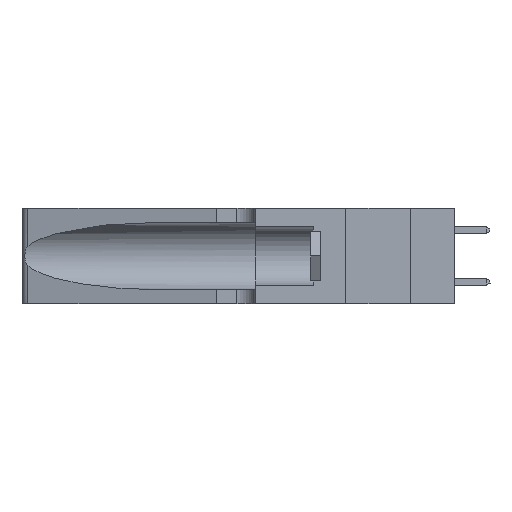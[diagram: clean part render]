
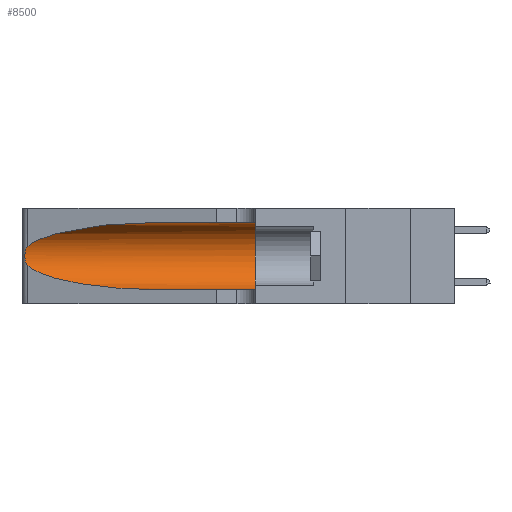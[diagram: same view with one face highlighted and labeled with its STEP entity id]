
A CAD part, left-side view. The second image highlights one B-rep face of the part: STEP entity #8500.
In plain terms, the highlighted cylindrical face has radius 3.308 mm (diameter 6.617 mm), a partial arc.
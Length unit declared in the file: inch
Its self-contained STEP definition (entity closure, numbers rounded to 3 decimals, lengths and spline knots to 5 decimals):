
#525 = CARTESIAN_POINT ( 'NONE',  ( 0.2373, 1.15595, 0.08982 ) ) ;
#903 = EDGE_CURVE ( 'NONE', #39769, #9896, #15293, .T. ) ;
#2294 = EDGE_CURVE ( 'NONE', #9896, #13112, #42863, .T. ) ;
#2593 = CARTESIAN_POINT ( 'NONE',  ( 0.1305, 0.35, 0.31525 ) ) ;
#2891 = EDGE_LOOP ( 'NONE', ( #29773, #40669, #41727, #10534, #13680, #7924 ) ) ;
#3011 = CARTESIAN_POINT ( 'NONE',  ( 0.25856, 1.23593, 0.16098 ) ) ;
#3863 = CARTESIAN_POINT ( 'NONE',  ( 0.1305, 0.72297, 0.05475 ) ) ;
#4471 = VECTOR ( 'NONE', #37388, 39.37008 ) ;
#4519 = AXIS2_PLACEMENT_3D ( 'NONE', #41123, #21231, #24622 ) ;
#4777 = FACE_OUTER_BOUND ( 'NONE', #2891, .T. ) ;
#4916 = CARTESIAN_POINT ( 'NONE',  ( 0.1305, 0.72297, 0.05475 ) ) ;
#6243 = CARTESIAN_POINT ( 'NONE',  ( 0.25487, 1.22718, 0.22369 ) ) ;
#6380 = CARTESIAN_POINT ( 'NONE',  ( 0.25639, 1.23186, 0.15144 ) ) ;
#7137 = DIRECTION ( 'NONE',  ( 0., -1., 0. ) ) ;
#7431 = CARTESIAN_POINT ( 'NONE',  ( 0.1305, 1.61858, 0.31525 ) ) ;
#7924 = ORIENTED_EDGE ( 'NONE', *, *, #27173, .F. ) ;
#8186 = EDGE_CURVE ( 'NONE', #14373, #39769, #42957, .T. ) ;
#8500 = ADVANCED_FACE ( 'NONE', ( #4777 ), #12662, .F. ) ;
#9625 = CARTESIAN_POINT ( 'NONE',  ( 0.25555, 1.22994, 0.2215 ) ) ;
#9757 = CARTESIAN_POINT ( 'NONE',  ( 0.25487, 1.22718, 0.14631 ) ) ;
#9896 = VERTEX_POINT ( 'NONE', #4916 ) ;
#10534 = ORIENTED_EDGE ( 'NONE', *, *, #2294, .T. ) ;
#12099 =( BOUNDED_CURVE ( )  B_SPLINE_CURVE ( 3, ( #35164, #38493, #18640, #41851 ),
 .UNSPECIFIED., .F., .F. ) 
 B_SPLINE_CURVE_WITH_KNOTS ( ( 4, 4 ),
 ( 1.5708, 2.84003 ),
 .UNSPECIFIED. ) 
 CURVE ( )  GEOMETRIC_REPRESENTATION_ITEM ( )  RATIONAL_B_SPLINE_CURVE ( ( 1., 0.87, 0.87, 1. ) ) 
 REPRESENTATION_ITEM ( '' )  );
#12662 = CYLINDRICAL_SURFACE ( 'NONE', #4519, 0.13025 ) ;
#12986 = CARTESIAN_POINT ( 'NONE',  ( 0.25639, 1.23184, 0.21858 ) ) ;
#13112 = VERTEX_POINT ( 'NONE', #34174 ) ;
#13680 = ORIENTED_EDGE ( 'NONE', *, *, #14604, .F. ) ;
#13877 = CARTESIAN_POINT ( 'NONE',  ( 0.1305, 1.61858, 0.05475 ) ) ;
#14373 = VERTEX_POINT ( 'NONE', #19945 ) ;
#14604 = EDGE_CURVE ( 'NONE', #42783, #13112, #31047, .T. ) ;
#15293 =( BOUNDED_CURVE ( )  B_SPLINE_CURVE ( 3, ( #40389, #525, #20532, #3863 ),
 .UNSPECIFIED., .F., .T. ) 
 B_SPLINE_CURVE_WITH_KNOTS ( ( 4, 4 ),
 ( 3.44316, 4.71239 ),
 .UNSPECIFIED. ) 
 CURVE ( )  GEOMETRIC_REPRESENTATION_ITEM ( )  RATIONAL_B_SPLINE_CURVE ( ( 1., 0.87, 0.87, 1. ) ) 
 REPRESENTATION_ITEM ( '' )  );
#16332 = CARTESIAN_POINT ( 'NONE',  ( 0.25854, 1.2359, 0.20912 ) ) ;
#17746 = CARTESIAN_POINT ( 'NONE',  ( 0.1305, 0.35, 0.185 ) ) ;
#18640 = CARTESIAN_POINT ( 'NONE',  ( 0.2373, 1.15595, 0.28018 ) ) ;
#19666 = CARTESIAN_POINT ( 'NONE',  ( 0.26075, 1.23896, 0.19203 ) ) ;
#19945 = CARTESIAN_POINT ( 'NONE',  ( 0.25487, 1.22718, 0.22369 ) ) ;
#20532 = CARTESIAN_POINT ( 'NONE',  ( 0.18966, 0.96281, 0.05475 ) ) ;
#21085 = DIRECTION ( 'NONE',  ( 0., 0., 1. ) ) ;
#21231 = DIRECTION ( 'NONE',  ( 0., -1., 0. ) ) ;
#21726 = AXIS2_PLACEMENT_3D ( 'NONE', #17746, #40956, #21085 ) ;
#21754 = CARTESIAN_POINT ( 'NONE',  ( 0.25487, 1.22718, 0.14631 ) ) ;
#23040 = CARTESIAN_POINT ( 'NONE',  ( 0.26017, 1.23833, 0.17102 ) ) ;
#24622 = DIRECTION ( 'NONE',  ( 0., 0., -1. ) ) ;
#26392 = CARTESIAN_POINT ( 'NONE',  ( 0.25789, 1.23486, 0.15765 ) ) ;
#27173 = EDGE_CURVE ( 'NONE', #42815, #42783, #39878, .T. ) ;
#29155 = EDGE_CURVE ( 'NONE', #42815, #14373, #12099, .T. ) ;
#29686 = CARTESIAN_POINT ( 'NONE',  ( 0.25555, 1.22993, 0.14849 ) ) ;
#29773 = ORIENTED_EDGE ( 'NONE', *, *, #29155, .T. ) ;
#31047 = CIRCLE ( 'NONE', #21726, 0.13025 ) ;
#32701 = CARTESIAN_POINT ( 'NONE',  ( 0.1305, 0.72297, 0.31525 ) ) ;
#34016 = VECTOR ( 'NONE', #7137, 39.37008 ) ;
#34174 = CARTESIAN_POINT ( 'NONE',  ( 0.1305, 0.35, 0.05475 ) ) ;
#35164 = CARTESIAN_POINT ( 'NONE',  ( 0.1305, 0.72297, 0.31525 ) ) ;
#36197 = CARTESIAN_POINT ( 'NONE',  ( 0.25787, 1.23484, 0.2124 ) ) ;
#37388 = DIRECTION ( 'NONE',  ( 0., -1., 0. ) ) ;
#38493 = CARTESIAN_POINT ( 'NONE',  ( 0.18966, 0.96281, 0.31525 ) ) ;
#39534 = CARTESIAN_POINT ( 'NONE',  ( 0.26018, 1.23835, 0.19895 ) ) ;
#39769 = VERTEX_POINT ( 'NONE', #21754 ) ;
#39878 = LINE ( 'NONE', #7431, #4471 ) ;
#40389 = CARTESIAN_POINT ( 'NONE',  ( 0.25487, 1.22718, 0.14631 ) ) ;
#40669 = ORIENTED_EDGE ( 'NONE', *, *, #8186, .T. ) ;
#40956 = DIRECTION ( 'NONE',  ( 0., 1., 0. ) ) ;
#41123 = CARTESIAN_POINT ( 'NONE',  ( 0.1305, 1.61858, 0.185 ) ) ;
#41727 = ORIENTED_EDGE ( 'NONE', *, *, #903, .T. ) ;
#41851 = CARTESIAN_POINT ( 'NONE',  ( 0.25487, 1.22718, 0.22369 ) ) ;
#42783 = VERTEX_POINT ( 'NONE', #2593 ) ;
#42815 = VERTEX_POINT ( 'NONE', #32701 ) ;
#42863 = LINE ( 'NONE', #13877, #34016 ) ;
#42869 = CARTESIAN_POINT ( 'NONE',  ( 0.26075, 1.23896, 0.178 ) ) ;
#42957 = B_SPLINE_CURVE_WITH_KNOTS ( 'NONE', 3,
 ( #6243, #9625, #12986, #36197, #16332, #39534, #19666, #42869, #23040, #3011, #26392, #6380, #29686, #9757 ),
 .UNSPECIFIED., .F., .F.,
 ( 4, 2, 2, 2, 2, 2, 4 ),
 ( 0., 0.00027, 0.00053, 0.00107, 0.0016, 0.00187, 0.00214 ),
 .UNSPECIFIED. ) ;
